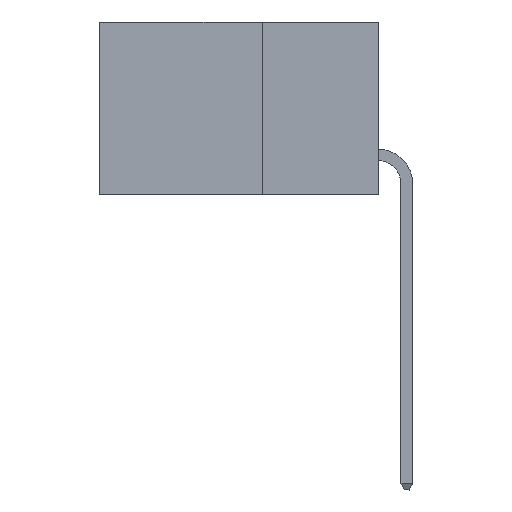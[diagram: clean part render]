
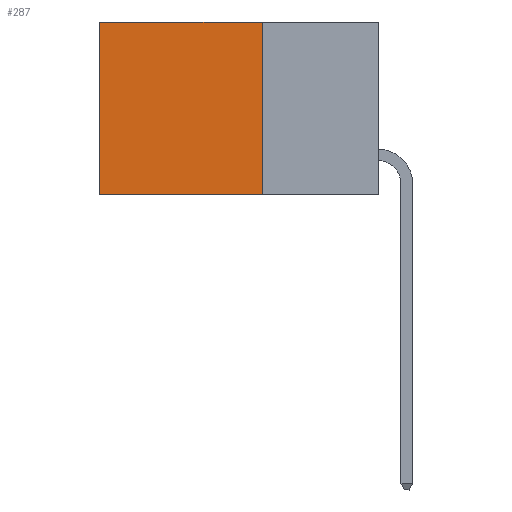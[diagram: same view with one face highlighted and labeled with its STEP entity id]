
A CAD part, left-side view. The second image highlights one B-rep face of the part: STEP entity #287.
In plain terms, the highlighted planar face has unit normal (-1, 0, 0).
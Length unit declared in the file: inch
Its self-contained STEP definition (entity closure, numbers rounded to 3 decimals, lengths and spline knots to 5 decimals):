
#100 = DIRECTION ( 'NONE',  ( 0., 1., 0. ) ) ;
#287 = ADVANCED_FACE ( 'NONE', ( #7260 ), #5007, .F. ) ;
#509 = ORIENTED_EDGE ( 'NONE', *, *, #16423, .F. ) ;
#571 = CARTESIAN_POINT ( 'NONE',  ( 0.298, 0.25, -0.37 ) ) ;
#1304 = AXIS2_PLACEMENT_3D ( 'NONE', #9180, #26055, #25789 ) ;
#1319 = LINE ( 'NONE', #16878, #3927 ) ;
#2144 = EDGE_CURVE ( 'NONE', #19544, #11538, #1319, .T. ) ;
#3187 = VECTOR ( 'NONE', #5808, 39.37008 ) ;
#3356 = EDGE_CURVE ( 'NONE', #15474, #25833, #10656, .T. ) ;
#3927 = VECTOR ( 'NONE', #6719, 39.37008 ) ;
#5007 = PLANE ( 'NONE',  #1304 ) ;
#5242 = ORIENTED_EDGE ( 'NONE', *, *, #2144, .F. ) ;
#5808 = DIRECTION ( 'NONE',  ( 0., 0., -1. ) ) ;
#6645 = DIRECTION ( 'NONE',  ( 0., 1., 0. ) ) ;
#6719 = DIRECTION ( 'NONE',  ( 0., 0., -1. ) ) ;
#7260 = FACE_OUTER_BOUND ( 'NONE', #14844, .T. ) ;
#9180 = CARTESIAN_POINT ( 'NONE',  ( 0.298, 0.25, 0. ) ) ;
#9264 = LINE ( 'NONE', #12379, #14188 ) ;
#10512 = ORIENTED_EDGE ( 'NONE', *, *, #18385, .T. ) ;
#10656 = LINE ( 'NONE', #18025, #3187 ) ;
#10807 = CARTESIAN_POINT ( 'NONE',  ( 0.298, 0.6, -0.37 ) ) ;
#10819 = CARTESIAN_POINT ( 'NONE',  ( 0.298, 0.25, -0.37 ) ) ;
#11538 = VERTEX_POINT ( 'NONE', #571 ) ;
#12379 = CARTESIAN_POINT ( 'NONE',  ( 0.298, 0.25, 0. ) ) ;
#14188 = VECTOR ( 'NONE', #100, 39.37008 ) ;
#14844 = EDGE_LOOP ( 'NONE', ( #20193, #509, #5242, #10512 ) ) ;
#15474 = VERTEX_POINT ( 'NONE', #21583 ) ;
#16423 = EDGE_CURVE ( 'NONE', #11538, #25833, #23025, .T. ) ;
#16878 = CARTESIAN_POINT ( 'NONE',  ( 0.298, 0.25, 0. ) ) ;
#17501 = VECTOR ( 'NONE', #6645, 39.37008 ) ;
#18025 = CARTESIAN_POINT ( 'NONE',  ( 0.298, 0.6, 0. ) ) ;
#18385 = EDGE_CURVE ( 'NONE', #19544, #15474, #9264, .T. ) ;
#19544 = VERTEX_POINT ( 'NONE', #26029 ) ;
#20193 = ORIENTED_EDGE ( 'NONE', *, *, #3356, .T. ) ;
#21583 = CARTESIAN_POINT ( 'NONE',  ( 0.298, 0.6, 0. ) ) ;
#23025 = LINE ( 'NONE', #10819, #17501 ) ;
#25789 = DIRECTION ( 'NONE',  ( 0., 0., -1. ) ) ;
#25833 = VERTEX_POINT ( 'NONE', #10807 ) ;
#26029 = CARTESIAN_POINT ( 'NONE',  ( 0.298, 0.25, 0. ) ) ;
#26055 = DIRECTION ( 'NONE',  ( 1., 0., 0. ) ) ;
